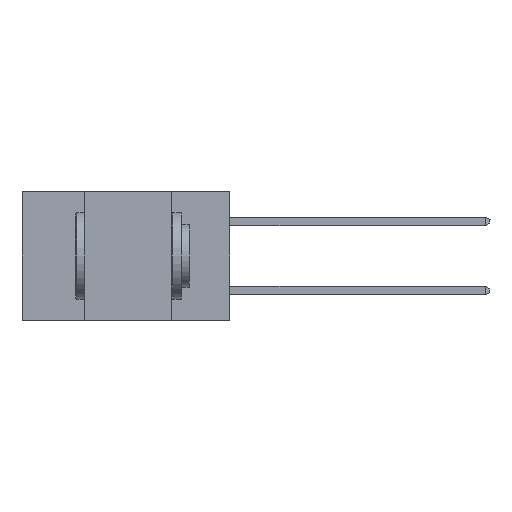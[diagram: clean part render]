
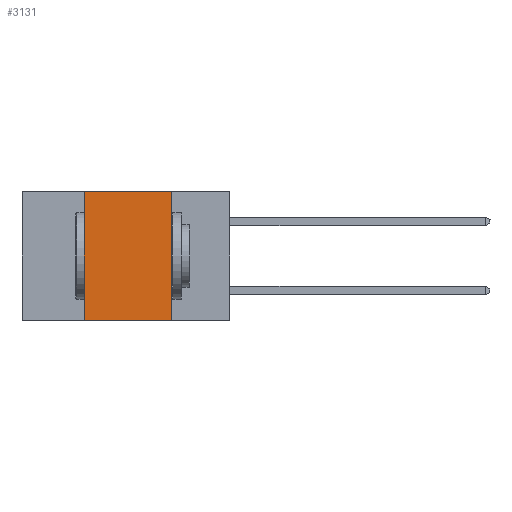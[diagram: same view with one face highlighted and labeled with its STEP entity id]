
A CAD part, left-side view. The second image highlights one B-rep face of the part: STEP entity #3131.
In plain terms, the highlighted planar face has unit normal (-1, 0, 0).
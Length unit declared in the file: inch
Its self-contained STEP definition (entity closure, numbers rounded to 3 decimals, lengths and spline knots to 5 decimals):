
#2256 = DIRECTION ( 'NONE',  ( 0., 0., -1. ) ) ;
#2442 = VECTOR ( 'NONE', #14711, 39.37008 ) ;
#2443 = EDGE_CURVE ( 'NONE', #13190, #5586, #20932, .T. ) ;
#2516 = VECTOR ( 'NONE', #18967, 39.37008 ) ;
#3097 = LINE ( 'NONE', #11187, #2516 ) ;
#3131 = ADVANCED_FACE ( 'NONE', ( #5852 ), #21968, .F. ) ;
#3806 = DIRECTION ( 'NONE',  ( 0., 0., -1. ) ) ;
#3971 = ORIENTED_EDGE ( 'NONE', *, *, #9644, .F. ) ;
#4748 = CARTESIAN_POINT ( 'NONE',  ( 0., 0.42, -0.37 ) ) ;
#5586 = VERTEX_POINT ( 'NONE', #19135 ) ;
#5852 = FACE_OUTER_BOUND ( 'NONE', #24989, .T. ) ;
#6659 = CARTESIAN_POINT ( 'NONE',  ( 0., 0.42, -0.37 ) ) ;
#6813 = AXIS2_PLACEMENT_3D ( 'NONE', #26065, #19993, #2256 ) ;
#7274 = CARTESIAN_POINT ( 'NONE',  ( 0., 0.17, 0. ) ) ;
#7847 = VECTOR ( 'NONE', #19796, 39.37008 ) ;
#9644 = EDGE_CURVE ( 'NONE', #15206, #16289, #17830, .T. ) ;
#9651 = EDGE_CURVE ( 'NONE', #13190, #16289, #18091, .T. ) ;
#10250 = ORIENTED_EDGE ( 'NONE', *, *, #9651, .T. ) ;
#11187 = CARTESIAN_POINT ( 'NONE',  ( 0., 0.6, 0. ) ) ;
#13190 = VERTEX_POINT ( 'NONE', #4748 ) ;
#14711 = DIRECTION ( 'NONE',  ( 0., 0., 1. ) ) ;
#15206 = VERTEX_POINT ( 'NONE', #7274 ) ;
#15426 = ORIENTED_EDGE ( 'NONE', *, *, #20935, .F. ) ;
#16289 = VERTEX_POINT ( 'NONE', #19973 ) ;
#17830 = LINE ( 'NONE', #20316, #19659 ) ;
#18091 = LINE ( 'NONE', #20066, #7847 ) ;
#18967 = DIRECTION ( 'NONE',  ( 0., -1., 0. ) ) ;
#19135 = CARTESIAN_POINT ( 'NONE',  ( 0., 0.42, 0. ) ) ;
#19659 = VECTOR ( 'NONE', #3806, 39.37008 ) ;
#19796 = DIRECTION ( 'NONE',  ( 0., -1., 0. ) ) ;
#19973 = CARTESIAN_POINT ( 'NONE',  ( 0., 0.17, -0.37 ) ) ;
#19993 = DIRECTION ( 'NONE',  ( 1., 0., 0. ) ) ;
#20066 = CARTESIAN_POINT ( 'NONE',  ( 0., 0.6, -0.37 ) ) ;
#20316 = CARTESIAN_POINT ( 'NONE',  ( 0., 0.17, -0.37 ) ) ;
#20932 = LINE ( 'NONE', #6659, #2442 ) ;
#20935 = EDGE_CURVE ( 'NONE', #5586, #15206, #3097, .T. ) ;
#21401 = ORIENTED_EDGE ( 'NONE', *, *, #2443, .F. ) ;
#21968 = PLANE ( 'NONE',  #6813 ) ;
#24989 = EDGE_LOOP ( 'NONE', ( #3971, #15426, #21401, #10250 ) ) ;
#26065 = CARTESIAN_POINT ( 'NONE',  ( 0., 0.6, 0. ) ) ;
